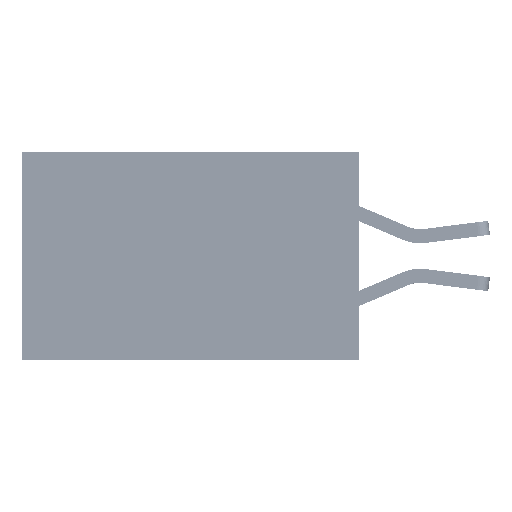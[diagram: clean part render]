
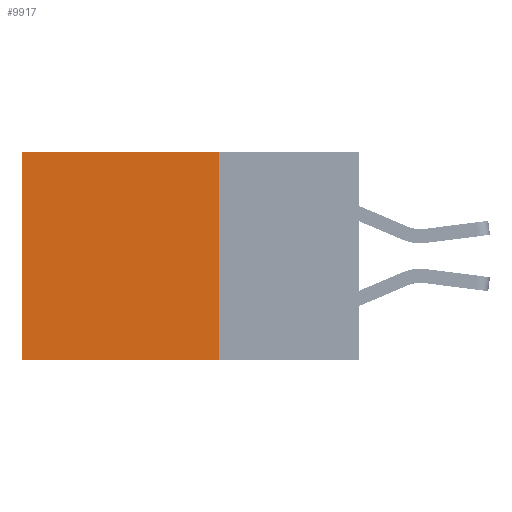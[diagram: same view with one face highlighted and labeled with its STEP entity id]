
A CAD part, left-side view. The second image highlights one B-rep face of the part: STEP entity #9917.
In plain terms, the highlighted planar face has unit normal (-1, 0, 0).
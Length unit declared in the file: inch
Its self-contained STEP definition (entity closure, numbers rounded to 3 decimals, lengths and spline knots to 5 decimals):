
#614 = DIRECTION ( 'NONE',  ( 0., 1., 0. ) ) ;
#2584 = VERTEX_POINT ( 'NONE', #28262 ) ;
#3256 = DIRECTION ( 'NONE',  ( 0., 0., -1. ) ) ;
#4609 = LINE ( 'NONE', #5354, #42005 ) ;
#5354 = CARTESIAN_POINT ( 'NONE',  ( 0.2875, 0.6, 0. ) ) ;
#5418 = CARTESIAN_POINT ( 'NONE',  ( 0.2875, 0.25, 0. ) ) ;
#6384 = PLANE ( 'NONE',  #24697 ) ;
#7544 = ORIENTED_EDGE ( 'NONE', *, *, #19856, .F. ) ;
#7761 = VERTEX_POINT ( 'NONE', #19364 ) ;
#9917 = ADVANCED_FACE ( 'NONE', ( #15522 ), #6384, .F. ) ;
#10011 = CARTESIAN_POINT ( 'NONE',  ( 0.2875, 0.25, 0. ) ) ;
#12272 = VECTOR ( 'NONE', #614, 39.37008 ) ;
#13296 = ORIENTED_EDGE ( 'NONE', *, *, #14340, .F. ) ;
#14340 = EDGE_CURVE ( 'NONE', #41435, #18455, #29777, .T. ) ;
#14980 = ORIENTED_EDGE ( 'NONE', *, *, #41754, .T. ) ;
#15522 = FACE_OUTER_BOUND ( 'NONE', #40039, .T. ) ;
#17626 = CARTESIAN_POINT ( 'NONE',  ( 0.2875, 0.25, 0. ) ) ;
#18455 = VERTEX_POINT ( 'NONE', #32592 ) ;
#19149 = VECTOR ( 'NONE', #3256, 39.37008 ) ;
#19364 = CARTESIAN_POINT ( 'NONE',  ( 0.2875, 0.6, 0. ) ) ;
#19856 = EDGE_CURVE ( 'NONE', #2584, #41435, #38430, .T. ) ;
#22152 = EDGE_CURVE ( 'NONE', #7761, #18455, #4609, .T. ) ;
#24697 = AXIS2_PLACEMENT_3D ( 'NONE', #10011, #45856, #27692 ) ;
#26507 = DIRECTION ( 'NONE',  ( 0., 0., -1. ) ) ;
#27010 = LINE ( 'NONE', #5418, #45293 ) ;
#27692 = DIRECTION ( 'NONE',  ( 0., 0., -1. ) ) ;
#28262 = CARTESIAN_POINT ( 'NONE',  ( 0.2875, 0.25, 0. ) ) ;
#29777 = LINE ( 'NONE', #30019, #12272 ) ;
#30019 = CARTESIAN_POINT ( 'NONE',  ( 0.2875, 0.25, -0.37 ) ) ;
#32592 = CARTESIAN_POINT ( 'NONE',  ( 0.2875, 0.6, -0.37 ) ) ;
#34055 = DIRECTION ( 'NONE',  ( 0., 1., 0. ) ) ;
#36951 = CARTESIAN_POINT ( 'NONE',  ( 0.2875, 0.25, -0.37 ) ) ;
#38430 = LINE ( 'NONE', #17626, #19149 ) ;
#40039 = EDGE_LOOP ( 'NONE', ( #40503, #13296, #7544, #14980 ) ) ;
#40503 = ORIENTED_EDGE ( 'NONE', *, *, #22152, .T. ) ;
#41435 = VERTEX_POINT ( 'NONE', #36951 ) ;
#41754 = EDGE_CURVE ( 'NONE', #2584, #7761, #27010, .T. ) ;
#42005 = VECTOR ( 'NONE', #26507, 39.37008 ) ;
#45293 = VECTOR ( 'NONE', #34055, 39.37008 ) ;
#45856 = DIRECTION ( 'NONE',  ( 1., 0., 0. ) ) ;
